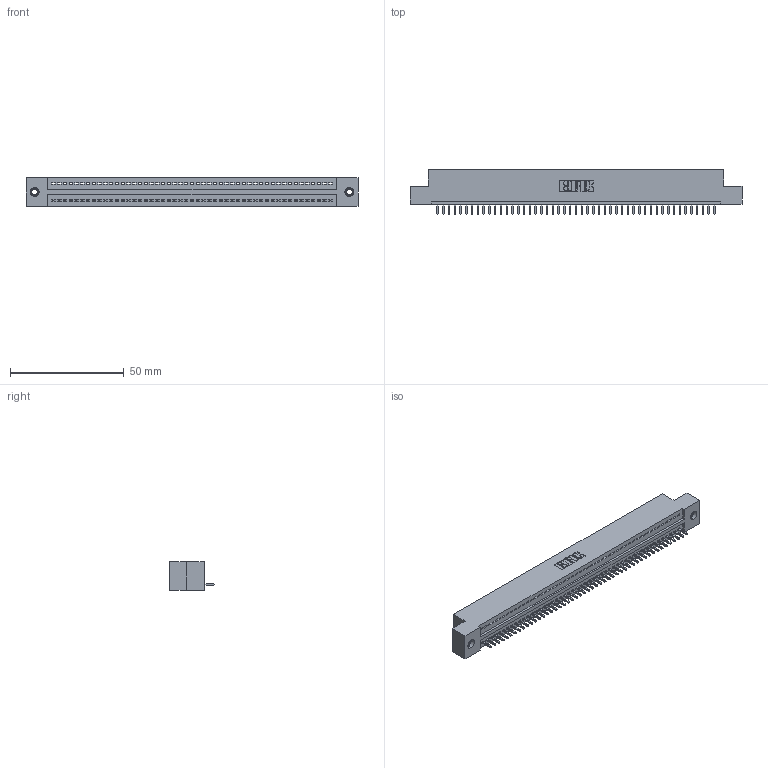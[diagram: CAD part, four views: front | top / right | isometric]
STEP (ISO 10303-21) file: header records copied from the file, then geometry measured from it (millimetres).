
FILE_DESCRIPTION (( 'STEP AP203' ), '1' );
FILE_NAME ('325-049-520-107.STEP', '2020-02-24T23:38:13', ( '' ), ( '' ), 'SwSTEP 2.0', 'SolidWorks 2016', '' );
FILE_SCHEMA (( 'CONFIG_CONTROL_DESIGN' ));
Length unit declared in the file: inch
Products named in the file (4): 325 Part_TI; 325-049-520-107; 325-292-001_325-293-120; 345-250-001_345-250-005-103
Assembly tree (52 placements, depth 2):
  325-049-520-107
    325 Part_TI
    325-292-001_325-293-120  x49
    345-250-001_345-250-005-103  x2
Bounding box: 146.18 x 19.68 x 12.45 mm (x, y, z)
Volume: 18472.1 mm3; surface area: 19811.5 mm2
Topology: 52 solids, 52 shells, 3016 faces, 9071 edges, 5974 vertices
Faces by surface type: plane 2160, cylinder 840, cone 12, torus 4
Entity records: 30254 total; most frequent: CARTESIAN_POINT 5200, ORIENTED_EDGE 5178, DIRECTION 4405, EDGE_CURVE 2589, LINE 2441, VECTOR 2441, VERTEX_POINT 1720, AXIS2_PLACEMENT_3D 982
